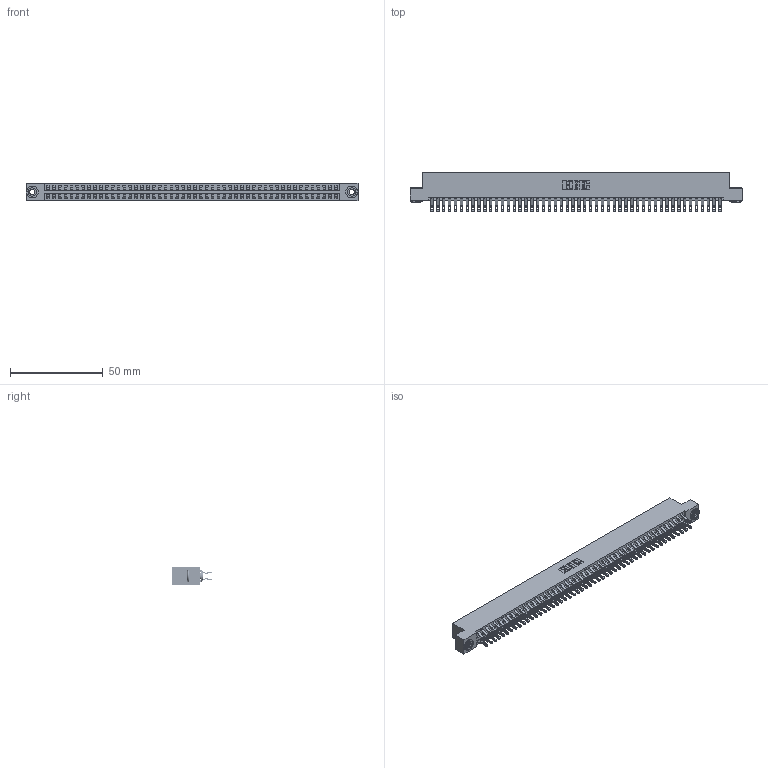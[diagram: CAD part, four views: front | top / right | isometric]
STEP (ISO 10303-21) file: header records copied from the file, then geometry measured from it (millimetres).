
FILE_DESCRIPTION (( 'STEP AP203' ), '1' );
FILE_NAME ('396-100-555-203.STEP', '2018-09-14T07:39:47', ( '' ), ( '' ), 'SwSTEP 2.0', 'SolidWorks 2016', '' );
FILE_SCHEMA (( 'CONFIG_CONTROL_DESIGN' ));
Length unit declared in the file: inch
Products named in the file (4): 346 Part_Flush Mounting Lugs - 0.156 Dia-TH; 345-292-001_555 Tail; 345-250-002_345-250-002-102; 396-100-555-203
Assembly tree (103 placements, depth 2):
  396-100-555-203
    346 Part_Flush Mounting Lugs - 0.156 Dia-TH
    345-292-001_555 Tail  x100
    345-250-002_345-250-002-102  x2
Bounding box: 179.32 x 21.46 x 9.4 mm (x, y, z)
Volume: 17857.9 mm3; surface area: 25920.7 mm2
Topology: 103 solids, 103 shells, 5960 faces, 18705 edges, 12466 vertices
Faces by surface type: plane 3386, cylinder 2566, cone 8
Entity records: 32530 total; most frequent: CARTESIAN_POINT 5361, ORIENTED_EDGE 5258, DIRECTION 4775, EDGE_CURVE 2629, VECTOR 2253, LINE 2253, VERTEX_POINT 1750, AXIS2_PLACEMENT_3D 1261
